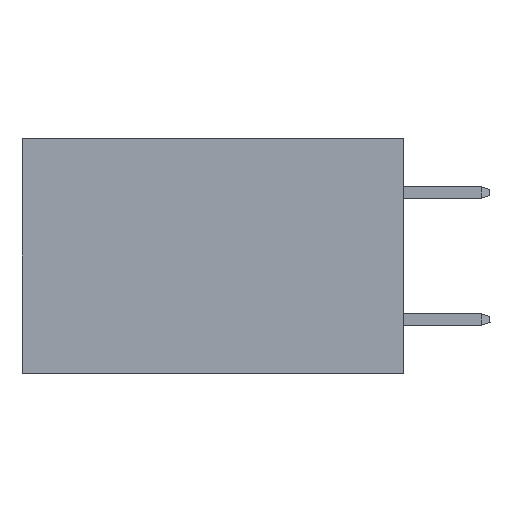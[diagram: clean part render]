
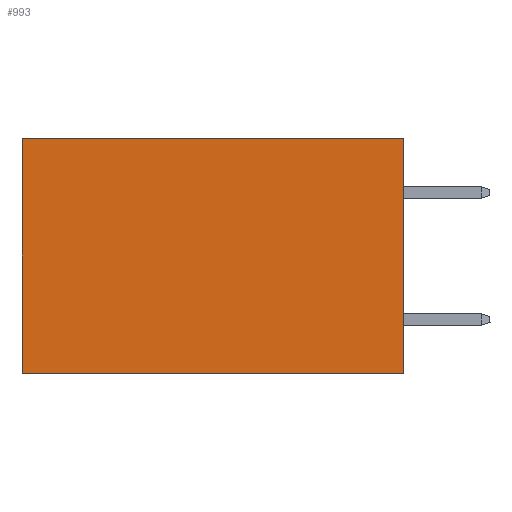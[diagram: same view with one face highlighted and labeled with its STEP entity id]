
A CAD part, left-side view. The second image highlights one B-rep face of the part: STEP entity #993.
In plain terms, the highlighted planar face has unit normal (-1, 0, 0).
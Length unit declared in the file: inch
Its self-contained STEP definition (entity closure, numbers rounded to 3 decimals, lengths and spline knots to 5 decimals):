
#773 = CARTESIAN_POINT ( 'NONE',  ( 0.2875, 0., 0. ) ) ;
#993 = ADVANCED_FACE ( 'NONE', ( #15324 ), #4472, .F. ) ;
#3177 = EDGE_CURVE ( 'NONE', #7149, #11979, #13357, .T. ) ;
#3590 = CARTESIAN_POINT ( 'NONE',  ( 0.2875, 0., 0. ) ) ;
#3935 = VECTOR ( 'NONE', #7008, 39.37008 ) ;
#4236 = EDGE_LOOP ( 'NONE', ( #15748, #20958, #6379, #17537 ) ) ;
#4472 = PLANE ( 'NONE',  #7820 ) ;
#4709 = LINE ( 'NONE', #18730, #19738 ) ;
#5026 = LINE ( 'NONE', #19373, #3935 ) ;
#6379 = ORIENTED_EDGE ( 'NONE', *, *, #3177, .F. ) ;
#6874 = VERTEX_POINT ( 'NONE', #19818 ) ;
#7008 = DIRECTION ( 'NONE',  ( 0., 1., 0. ) ) ;
#7149 = VERTEX_POINT ( 'NONE', #3590 ) ;
#7820 = AXIS2_PLACEMENT_3D ( 'NONE', #9860, #16934, #17173 ) ;
#7874 = DIRECTION ( 'NONE',  ( 0., 0., -1. ) ) ;
#7991 = DIRECTION ( 'NONE',  ( 0., 0., -1. ) ) ;
#9860 = CARTESIAN_POINT ( 'NONE',  ( 0.2875, 0., 0. ) ) ;
#10678 = EDGE_CURVE ( 'NONE', #19173, #6874, #13237, .T. ) ;
#11979 = VERTEX_POINT ( 'NONE', #17722 ) ;
#11991 = CARTESIAN_POINT ( 'NONE',  ( 0.2875, 0.6, 0. ) ) ;
#13237 = LINE ( 'NONE', #13483, #16060 ) ;
#13357 = LINE ( 'NONE', #773, #21943 ) ;
#13483 = CARTESIAN_POINT ( 'NONE',  ( 0.2875, 0.6, 0. ) ) ;
#15324 = FACE_OUTER_BOUND ( 'NONE', #4236, .T. ) ;
#15748 = ORIENTED_EDGE ( 'NONE', *, *, #10678, .T. ) ;
#16060 = VECTOR ( 'NONE', #7991, 39.37008 ) ;
#16934 = DIRECTION ( 'NONE',  ( 1., 0., 0. ) ) ;
#17173 = DIRECTION ( 'NONE',  ( 0., 0., -1. ) ) ;
#17490 = EDGE_CURVE ( 'NONE', #7149, #19173, #5026, .T. ) ;
#17537 = ORIENTED_EDGE ( 'NONE', *, *, #17490, .T. ) ;
#17722 = CARTESIAN_POINT ( 'NONE',  ( 0.2875, 0., -0.37 ) ) ;
#18730 = CARTESIAN_POINT ( 'NONE',  ( 0.2875, 0., -0.37 ) ) ;
#19173 = VERTEX_POINT ( 'NONE', #11991 ) ;
#19373 = CARTESIAN_POINT ( 'NONE',  ( 0.2875, 0., 0. ) ) ;
#19738 = VECTOR ( 'NONE', #20682, 39.37008 ) ;
#19818 = CARTESIAN_POINT ( 'NONE',  ( 0.2875, 0.6, -0.37 ) ) ;
#20682 = DIRECTION ( 'NONE',  ( 0., 1., 0. ) ) ;
#20958 = ORIENTED_EDGE ( 'NONE', *, *, #22805, .F. ) ;
#21943 = VECTOR ( 'NONE', #7874, 39.37008 ) ;
#22805 = EDGE_CURVE ( 'NONE', #11979, #6874, #4709, .T. ) ;
